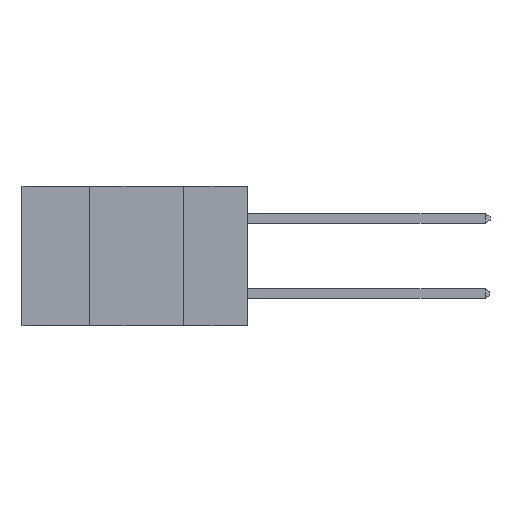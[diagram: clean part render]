
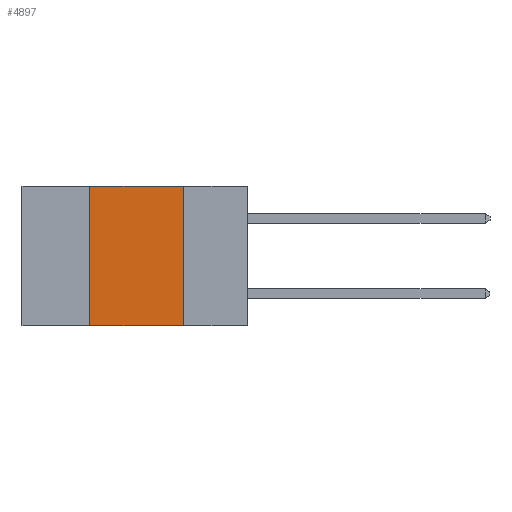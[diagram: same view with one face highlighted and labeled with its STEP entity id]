
A CAD part, left-side view. The second image highlights one B-rep face of the part: STEP entity #4897.
In plain terms, the highlighted planar face has unit normal (-1, 0, 0).
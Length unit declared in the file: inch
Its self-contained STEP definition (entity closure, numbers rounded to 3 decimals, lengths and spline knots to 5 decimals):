
#190 = EDGE_CURVE ( 'NONE', #17583, #13677, #4021, .T. ) ;
#2555 = ORIENTED_EDGE ( 'NONE', *, *, #20587, .F. ) ;
#2888 = CARTESIAN_POINT ( 'NONE',  ( 0., 0.42, 0. ) ) ;
#3630 = VECTOR ( 'NONE', #7885, 39.37008 ) ;
#4021 = LINE ( 'NONE', #24132, #16364 ) ;
#4897 = ADVANCED_FACE ( 'NONE', ( #26861 ), #10929, .F. ) ;
#7034 = EDGE_LOOP ( 'NONE', ( #12962, #13765, #2555, #15315 ) ) ;
#7885 = DIRECTION ( 'NONE',  ( 0., 0., 1. ) ) ;
#9617 = VERTEX_POINT ( 'NONE', #10252 ) ;
#10252 = CARTESIAN_POINT ( 'NONE',  ( 0., 0.17, 0. ) ) ;
#10289 = CARTESIAN_POINT ( 'NONE',  ( 0., 0.42, -0.37 ) ) ;
#10929 = PLANE ( 'NONE',  #12274 ) ;
#11080 = VECTOR ( 'NONE', #11099, 39.37008 ) ;
#11099 = DIRECTION ( 'NONE',  ( 0., 0., -1. ) ) ;
#12274 = AXIS2_PLACEMENT_3D ( 'NONE', #18257, #28211, #13404 ) ;
#12962 = ORIENTED_EDGE ( 'NONE', *, *, #15012, .F. ) ;
#13384 = EDGE_CURVE ( 'NONE', #24576, #9617, #17262, .T. ) ;
#13404 = DIRECTION ( 'NONE',  ( 0., 0., -1. ) ) ;
#13677 = VERTEX_POINT ( 'NONE', #30826 ) ;
#13765 = ORIENTED_EDGE ( 'NONE', *, *, #13384, .F. ) ;
#14829 = DIRECTION ( 'NONE',  ( 0., -1., 0. ) ) ;
#15012 = EDGE_CURVE ( 'NONE', #9617, #13677, #23397, .T. ) ;
#15315 = ORIENTED_EDGE ( 'NONE', *, *, #190, .T. ) ;
#15809 = CARTESIAN_POINT ( 'NONE',  ( 0., 0.42, 0. ) ) ;
#16364 = VECTOR ( 'NONE', #22855, 39.37008 ) ;
#17262 = LINE ( 'NONE', #19792, #28906 ) ;
#17583 = VERTEX_POINT ( 'NONE', #10289 ) ;
#18257 = CARTESIAN_POINT ( 'NONE',  ( 0., 0.6, 0. ) ) ;
#19792 = CARTESIAN_POINT ( 'NONE',  ( 0., 0.6, 0. ) ) ;
#20587 = EDGE_CURVE ( 'NONE', #17583, #24576, #23308, .T. ) ;
#22855 = DIRECTION ( 'NONE',  ( 0., -1., 0. ) ) ;
#23308 = LINE ( 'NONE', #2888, #3630 ) ;
#23397 = LINE ( 'NONE', #28370, #11080 ) ;
#24132 = CARTESIAN_POINT ( 'NONE',  ( 0., 0.6, -0.37 ) ) ;
#24576 = VERTEX_POINT ( 'NONE', #15809 ) ;
#26861 = FACE_OUTER_BOUND ( 'NONE', #7034, .T. ) ;
#28211 = DIRECTION ( 'NONE',  ( 1., 0., 0. ) ) ;
#28370 = CARTESIAN_POINT ( 'NONE',  ( 0., 0.17, 0. ) ) ;
#28906 = VECTOR ( 'NONE', #14829, 39.37008 ) ;
#30826 = CARTESIAN_POINT ( 'NONE',  ( 0., 0.17, -0.37 ) ) ;
